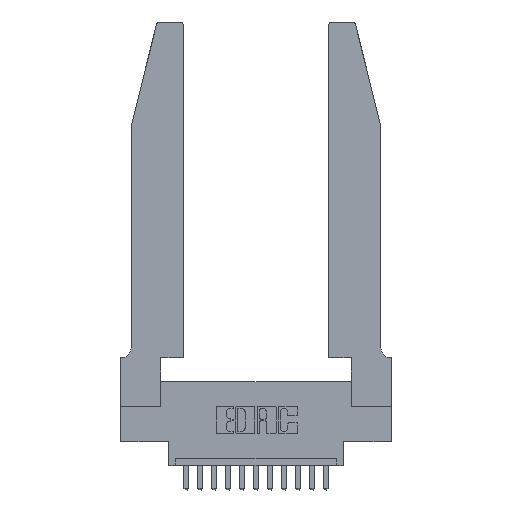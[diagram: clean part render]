
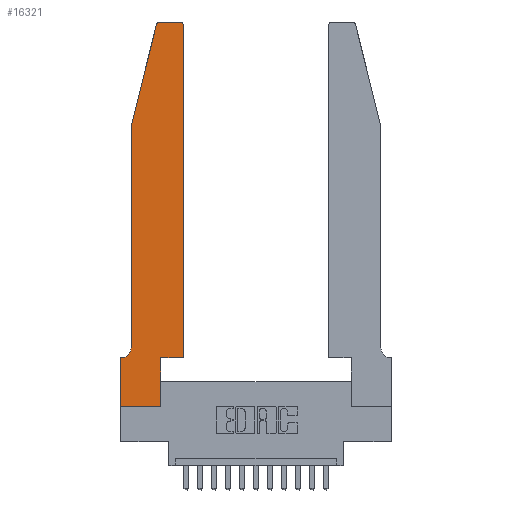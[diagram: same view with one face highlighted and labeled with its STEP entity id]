
A CAD part, top view. The second image highlights one B-rep face of the part: STEP entity #16321.
In plain terms, the highlighted planar face has unit normal (0, 0, 1).
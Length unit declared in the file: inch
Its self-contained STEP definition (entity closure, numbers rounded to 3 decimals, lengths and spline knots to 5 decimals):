
#219 = ORIENTED_EDGE ( 'NONE', *, *, #6920, .T. ) ;
#525 = LINE ( 'NONE', #17004, #16960 ) ;
#577 = ORIENTED_EDGE ( 'NONE', *, *, #5572, .T. ) ;
#578 = CARTESIAN_POINT ( 'NONE',  ( 0.284, 2.75, 0.37 ) ) ;
#709 = DIRECTION ( 'NONE',  ( 1., 0., 0. ) ) ;
#895 = ORIENTED_EDGE ( 'NONE', *, *, #8832, .T. ) ;
#1096 = CIRCLE ( 'NONE', #16029, 0.03 ) ;
#1106 = FACE_OUTER_BOUND ( 'NONE', #15800, .T. ) ;
#1459 = VECTOR ( 'NONE', #12737, 39.37008 ) ;
#1958 = ORIENTED_EDGE ( 'NONE', *, *, #12407, .T. ) ;
#2035 = VERTEX_POINT ( 'NONE', #9516 ) ;
#2103 = DIRECTION ( 'NONE',  ( 1., 0., 0. ) ) ;
#2119 = VECTOR ( 'NONE', #9406, 39.37008 ) ;
#2237 = EDGE_CURVE ( 'NONE', #10007, #5282, #1096, .T. ) ;
#2293 = VERTEX_POINT ( 'NONE', #11789 ) ;
#2759 = CARTESIAN_POINT ( 'NONE',  ( 0.4505, 0.35, 0.37 ) ) ;
#2969 = EDGE_CURVE ( 'NONE', #3130, #7264, #17091, .T. ) ;
#3130 = VERTEX_POINT ( 'NONE', #13914 ) ;
#3258 = DIRECTION ( 'NONE',  ( -1., 0., 0. ) ) ;
#3376 = PLANE ( 'NONE',  #12549 ) ;
#3465 = CARTESIAN_POINT ( 'NONE',  ( 0., 0.35, 0.37 ) ) ;
#3652 = DIRECTION ( 'NONE',  ( 1., 0., 0. ) ) ;
#3745 = DIRECTION ( 'NONE',  ( 0., -1., 0. ) ) ;
#4100 = VERTEX_POINT ( 'NONE', #7151 ) ;
#4143 = LINE ( 'NONE', #13166, #14460 ) ;
#4373 = VERTEX_POINT ( 'NONE', #5148 ) ;
#4841 = DIRECTION ( 'NONE',  ( 0., 0., 1. ) ) ;
#4974 = DIRECTION ( 'NONE',  ( 0., 1., 0. ) ) ;
#5148 = CARTESIAN_POINT ( 'NONE',  ( 0.4505, 2.72, 0.37 ) ) ;
#5257 = LINE ( 'NONE', #16364, #2119 ) ;
#5282 = VERTEX_POINT ( 'NONE', #13778 ) ;
#5572 = EDGE_CURVE ( 'NONE', #2035, #7101, #5257, .T. ) ;
#5888 = ORIENTED_EDGE ( 'NONE', *, *, #11682, .T. ) ;
#6046 = EDGE_CURVE ( 'NONE', #5282, #6824, #9263, .T. ) ;
#6731 = CARTESIAN_POINT ( 'NONE',  ( 0.0755, 2., 0.37 ) ) ;
#6824 = VERTEX_POINT ( 'NONE', #10296 ) ;
#6834 = EDGE_CURVE ( 'NONE', #6824, #4100, #14283, .T. ) ;
#6920 = EDGE_CURVE ( 'NONE', #4373, #2293, #7822, .T. ) ;
#7074 = AXIS2_PLACEMENT_3D ( 'NONE', #14652, #16039, #7999 ) ;
#7101 = VERTEX_POINT ( 'NONE', #3465 ) ;
#7151 = CARTESIAN_POINT ( 'NONE',  ( 0.0755, 0.42, 0.37 ) ) ;
#7264 = VERTEX_POINT ( 'NONE', #14541 ) ;
#7465 = ORIENTED_EDGE ( 'NONE', *, *, #9668, .T. ) ;
#7822 = CIRCLE ( 'NONE', #7074, 0.03 ) ;
#7999 = DIRECTION ( 'NONE',  ( 1., 0., 0. ) ) ;
#8832 = EDGE_CURVE ( 'NONE', #7101, #3130, #13573, .T. ) ;
#8868 = VECTOR ( 'NONE', #14595, 39.37008 ) ;
#8901 = VECTOR ( 'NONE', #3652, 39.37008 ) ;
#9263 = LINE ( 'NONE', #9641, #17274 ) ;
#9277 = DIRECTION ( 'NONE',  ( 0., 1., 0. ) ) ;
#9406 = DIRECTION ( 'NONE',  ( -1., 0., 0. ) ) ;
#9516 = CARTESIAN_POINT ( 'NONE',  ( 0.0055, 0.35, 0.37 ) ) ;
#9641 = CARTESIAN_POINT ( 'NONE',  ( 0.0755, 2., 0.37 ) ) ;
#9668 = EDGE_CURVE ( 'NONE', #4100, #2035, #13232, .T. ) ;
#9888 = CARTESIAN_POINT ( 'NONE',  ( 0.2865, 0.35, 0.37 ) ) ;
#10007 = VERTEX_POINT ( 'NONE', #578 ) ;
#10060 = CARTESIAN_POINT ( 'NONE',  ( 0.2605, 2.75, 0.37 ) ) ;
#10062 = CARTESIAN_POINT ( 'NONE',  ( 0.4505, 0.35, 0.37 ) ) ;
#10144 = CARTESIAN_POINT ( 'NONE',  ( 0., 0.35, 0.37 ) ) ;
#10221 = CARTESIAN_POINT ( 'NONE',  ( 0.284, 2.72, 0.37 ) ) ;
#10268 = EDGE_CURVE ( 'NONE', #2293, #10007, #13882, .T. ) ;
#10296 = CARTESIAN_POINT ( 'NONE',  ( 0.0755, 2., 0.37 ) ) ;
#10612 = VERTEX_POINT ( 'NONE', #10062 ) ;
#11128 = AXIS2_PLACEMENT_3D ( 'NONE', #16803, #12621, #3258 ) ;
#11519 = CARTESIAN_POINT ( 'NONE',  ( 0., 0., 0.37 ) ) ;
#11555 = ORIENTED_EDGE ( 'NONE', *, *, #2237, .T. ) ;
#11565 = DIRECTION ( 'NONE',  ( 0., 0., 1. ) ) ;
#11614 = CARTESIAN_POINT ( 'NONE',  ( 0., 0., 0.37 ) ) ;
#11682 = EDGE_CURVE ( 'NONE', #10612, #4373, #4143, .T. ) ;
#11757 = ORIENTED_EDGE ( 'NONE', *, *, #6834, .T. ) ;
#11789 = CARTESIAN_POINT ( 'NONE',  ( 0.4205, 2.75, 0.37 ) ) ;
#11804 = ORIENTED_EDGE ( 'NONE', *, *, #10268, .T. ) ;
#11879 = VECTOR ( 'NONE', #3745, 39.37008 ) ;
#12059 = ORIENTED_EDGE ( 'NONE', *, *, #2969, .T. ) ;
#12407 = EDGE_CURVE ( 'NONE', #13588, #10612, #16997, .T. ) ;
#12549 = AXIS2_PLACEMENT_3D ( 'NONE', #10144, #4841, #2103 ) ;
#12577 = ORIENTED_EDGE ( 'NONE', *, *, #6046, .T. ) ;
#12621 = DIRECTION ( 'NONE',  ( 0., 0., -1. ) ) ;
#12737 = DIRECTION ( 'NONE',  ( -1., 0., 0. ) ) ;
#13166 = CARTESIAN_POINT ( 'NONE',  ( 0.4505, 0.35, 0.37 ) ) ;
#13232 = CIRCLE ( 'NONE', #11128, 0.07 ) ;
#13293 = EDGE_CURVE ( 'NONE', #7264, #13588, #525, .T. ) ;
#13326 = DIRECTION ( 'NONE',  ( 1., 0., 0. ) ) ;
#13573 = LINE ( 'NONE', #11614, #11879 ) ;
#13588 = VERTEX_POINT ( 'NONE', #9888 ) ;
#13778 = CARTESIAN_POINT ( 'NONE',  ( 0.25487, 2.72718, 0.37 ) ) ;
#13882 = LINE ( 'NONE', #10060, #1459 ) ;
#13914 = CARTESIAN_POINT ( 'NONE',  ( 0., 0., 0.37 ) ) ;
#14283 = LINE ( 'NONE', #6731, #8868 ) ;
#14460 = VECTOR ( 'NONE', #9277, 39.37008 ) ;
#14541 = CARTESIAN_POINT ( 'NONE',  ( 0.2865, 0., 0.37 ) ) ;
#14595 = DIRECTION ( 'NONE',  ( 0., -1., 0. ) ) ;
#14652 = CARTESIAN_POINT ( 'NONE',  ( 0.4205, 2.72, 0.37 ) ) ;
#15062 = DIRECTION ( 'NONE',  ( -0.239, -0.971, 0. ) ) ;
#15779 = ORIENTED_EDGE ( 'NONE', *, *, #13293, .T. ) ;
#15800 = EDGE_LOOP ( 'NONE', ( #11804, #11555, #12577, #11757, #7465, #577, #895, #12059, #15779, #1958, #5888, #219 ) ) ;
#15949 = VECTOR ( 'NONE', #13326, 39.37008 ) ;
#16029 = AXIS2_PLACEMENT_3D ( 'NONE', #10221, #11565, #709 ) ;
#16039 = DIRECTION ( 'NONE',  ( 0., 0., 1. ) ) ;
#16321 = ADVANCED_FACE ( 'NONE', ( #1106 ), #3376, .T. ) ;
#16364 = CARTESIAN_POINT ( 'NONE',  ( 0.0755, 0.35, 0.37 ) ) ;
#16803 = CARTESIAN_POINT ( 'NONE',  ( 0.0055, 0.42, 0.37 ) ) ;
#16960 = VECTOR ( 'NONE', #4974, 39.37008 ) ;
#16997 = LINE ( 'NONE', #2759, #15949 ) ;
#17004 = CARTESIAN_POINT ( 'NONE',  ( 0.2865, 0.35, 0.37 ) ) ;
#17091 = LINE ( 'NONE', #11519, #8901 ) ;
#17274 = VECTOR ( 'NONE', #15062, 39.37008 ) ;
